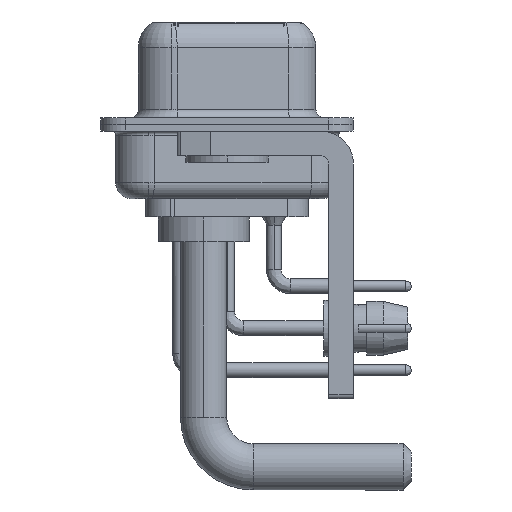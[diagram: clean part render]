
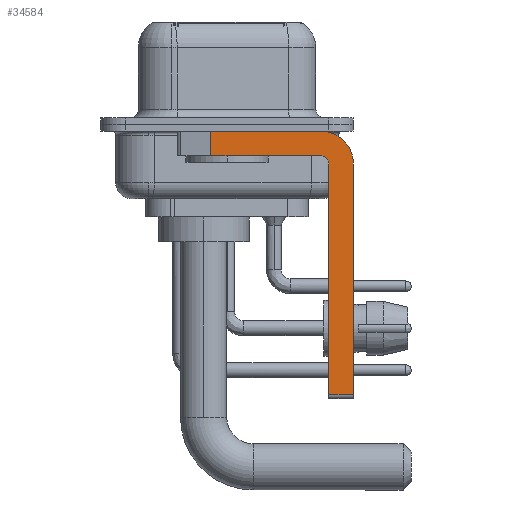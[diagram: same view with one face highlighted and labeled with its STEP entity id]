
A CAD part, left-side view. The second image highlights one B-rep face of the part: STEP entity #34584.
In plain terms, the highlighted planar face has unit normal (-1, 0, 0).
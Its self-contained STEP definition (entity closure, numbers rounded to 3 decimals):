
#261 = CARTESIAN_POINT ( 'NONE',  ( -2.9, -5.65, -16.35 ) ) ;
#313 = CARTESIAN_POINT ( 'NONE',  ( -2.9, -6.15, -2.4 ) ) ;
#357 = CARTESIAN_POINT ( 'NONE',  ( -2.9, 3., -0.4 ) ) ;
#410 = VECTOR ( 'NONE', #1601, 1000. ) ;
#466 = EDGE_CURVE ( 'NONE', #22084, #25347, #15199, .T. ) ;
#1601 = DIRECTION ( 'NONE',  ( 0., 0., 1. ) ) ;
#2057 = CIRCLE ( 'NONE', #17856, 0.5 ) ;
#2471 = EDGE_CURVE ( 'NONE', #25347, #21108, #2057, .T. ) ;
#3892 = DIRECTION ( 'NONE',  ( 1., 0., 0. ) ) ;
#4295 = ORIENTED_EDGE ( 'NONE', *, *, #16888, .F. ) ;
#5117 = LINE ( 'NONE', #357, #34922 ) ;
#5466 = DIRECTION ( 'NONE',  ( 0., 0., 1. ) ) ;
#6478 = DIRECTION ( 'NONE',  ( 0., 1., 0. ) ) ;
#6827 = CARTESIAN_POINT ( 'NONE',  ( -2.9, -5.65, -1.9 ) ) ;
#8209 = CARTESIAN_POINT ( 'NONE',  ( -2.9, -7.65, -2.4 ) ) ;
#8738 = AXIS2_PLACEMENT_3D ( 'NONE', #32579, #21776, #19141 ) ;
#9359 = PLANE ( 'NONE',  #11245 ) ;
#10491 = VECTOR ( 'NONE', #30677, 1000. ) ;
#10660 = CARTESIAN_POINT ( 'NONE',  ( -2.9, -7.65, -16.35 ) ) ;
#11245 = AXIS2_PLACEMENT_3D ( 'NONE', #28064, #3892, #14652 ) ;
#11752 = ORIENTED_EDGE ( 'NONE', *, *, #34383, .F. ) ;
#12011 = VERTEX_POINT ( 'NONE', #22222 ) ;
#12759 = ORIENTED_EDGE ( 'NONE', *, *, #30257, .T. ) ;
#12767 = VERTEX_POINT ( 'NONE', #10660 ) ;
#14652 = DIRECTION ( 'NONE',  ( 0., 0., -1. ) ) ;
#15199 = LINE ( 'NONE', #28610, #410 ) ;
#15357 = VERTEX_POINT ( 'NONE', #34899 ) ;
#16692 = DIRECTION ( 'NONE',  ( 0., -1., 0. ) ) ;
#16888 = EDGE_CURVE ( 'NONE', #21108, #12011, #31038, .T. ) ;
#17290 = FACE_OUTER_BOUND ( 'NONE', #22806, .T. ) ;
#17417 = CARTESIAN_POINT ( 'NONE',  ( -2.9, -5.65, -1.9 ) ) ;
#17616 = ORIENTED_EDGE ( 'NONE', *, *, #2471, .F. ) ;
#17856 = AXIS2_PLACEMENT_3D ( 'NONE', #21177, #29680, #5466 ) ;
#17881 = CARTESIAN_POINT ( 'NONE',  ( -2.9, 0.978, -0.4 ) ) ;
#19141 = DIRECTION ( 'NONE',  ( 0., 0., -1. ) ) ;
#19836 = ORIENTED_EDGE ( 'NONE', *, *, #29300, .F. ) ;
#21108 = VERTEX_POINT ( 'NONE', #17417 ) ;
#21177 = CARTESIAN_POINT ( 'NONE',  ( -2.9, -5.65, -2.4 ) ) ;
#21696 = LINE ( 'NONE', #32498, #10491 ) ;
#21776 = DIRECTION ( 'NONE',  ( 1., 0., 0. ) ) ;
#21819 = VERTEX_POINT ( 'NONE', #17881 ) ;
#22084 = VERTEX_POINT ( 'NONE', #33588 ) ;
#22222 = CARTESIAN_POINT ( 'NONE',  ( -2.9, 0.978, -1.9 ) ) ;
#22739 = EDGE_CURVE ( 'NONE', #22084, #12767, #24445, .T. ) ;
#22806 = EDGE_LOOP ( 'NONE', ( #11752, #12759, #4295, #17616, #22808, #27037, #31206, #19836 ) ) ;
#22808 = ORIENTED_EDGE ( 'NONE', *, *, #466, .F. ) ;
#23411 = VECTOR ( 'NONE', #27081, 1000. ) ;
#24445 = LINE ( 'NONE', #261, #30388 ) ;
#25347 = VERTEX_POINT ( 'NONE', #313 ) ;
#25353 = CARTESIAN_POINT ( 'NONE',  ( -2.9, -7.65, -2.4 ) ) ;
#27037 = ORIENTED_EDGE ( 'NONE', *, *, #22739, .T. ) ;
#27081 = DIRECTION ( 'NONE',  ( 0., 0., -1. ) ) ;
#28064 = CARTESIAN_POINT ( 'NONE',  ( -2.9, -5.65, -2.4 ) ) ;
#28610 = CARTESIAN_POINT ( 'NONE',  ( -2.9, -6.15, -16.6 ) ) ;
#29028 = CIRCLE ( 'NONE', #8738, 2. ) ;
#29300 = EDGE_CURVE ( 'NONE', #15357, #30193, #29028, .T. ) ;
#29680 = DIRECTION ( 'NONE',  ( -1., 0., 0. ) ) ;
#30193 = VERTEX_POINT ( 'NONE', #25353 ) ;
#30257 = EDGE_CURVE ( 'NONE', #21819, #12011, #21696, .T. ) ;
#30388 = VECTOR ( 'NONE', #16692, 1000. ) ;
#30513 = EDGE_CURVE ( 'NONE', #30193, #12767, #32409, .T. ) ;
#30677 = DIRECTION ( 'NONE',  ( 0., 0., -1. ) ) ;
#31038 = LINE ( 'NONE', #6827, #33029 ) ;
#31206 = ORIENTED_EDGE ( 'NONE', *, *, #30513, .F. ) ;
#31984 = DIRECTION ( 'NONE',  ( 0., -1., 0. ) ) ;
#32409 = LINE ( 'NONE', #8209, #23411 ) ;
#32498 = CARTESIAN_POINT ( 'NONE',  ( -2.9, 0.978, -1.9 ) ) ;
#32579 = CARTESIAN_POINT ( 'NONE',  ( -2.9, -5.65, -2.4 ) ) ;
#33029 = VECTOR ( 'NONE', #6478, 1000. ) ;
#33588 = CARTESIAN_POINT ( 'NONE',  ( -2.9, -6.15, -16.35 ) ) ;
#34383 = EDGE_CURVE ( 'NONE', #21819, #15357, #5117, .T. ) ;
#34584 = ADVANCED_FACE ( 'NONE', ( #17290 ), #9359, .F. ) ;
#34899 = CARTESIAN_POINT ( 'NONE',  ( -2.9, -5.65, -0.4 ) ) ;
#34922 = VECTOR ( 'NONE', #31984, 1000. ) ;
